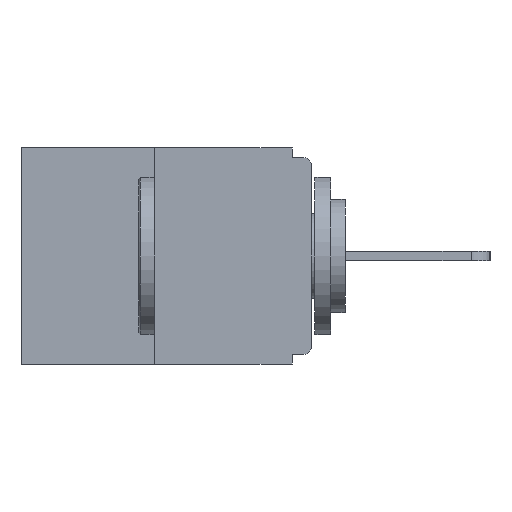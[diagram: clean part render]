
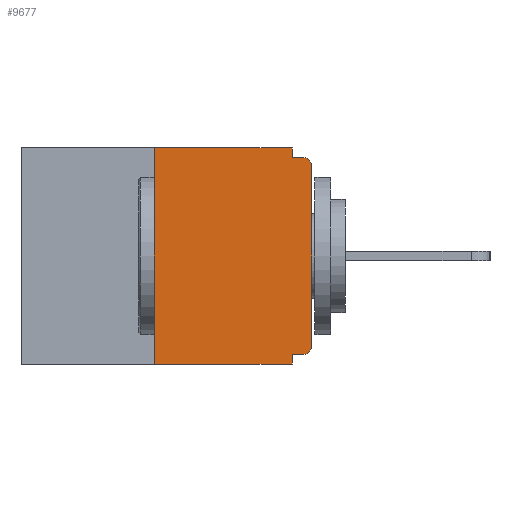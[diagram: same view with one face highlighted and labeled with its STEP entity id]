
A CAD part, left-side view. The second image highlights one B-rep face of the part: STEP entity #9677.
In plain terms, the highlighted planar face has unit normal (-1, 0, 0).
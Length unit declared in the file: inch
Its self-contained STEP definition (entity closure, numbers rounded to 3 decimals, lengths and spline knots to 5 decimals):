
#5 = VECTOR ( 'NONE', #2524, 39.37008 ) ;
#201 = VECTOR ( 'NONE', #8029, 39.37008 ) ;
#351 = EDGE_LOOP ( 'NONE', ( #2896, #9992, #2501, #7942, #8920, #2768, #10894, #2540, #6096, #4621 ) ) ;
#425 = LINE ( 'NONE', #11037, #5 ) ;
#451 = DIRECTION ( 'NONE',  ( 0., -1., 0. ) ) ;
#469 = FACE_OUTER_BOUND ( 'NONE', #351, .T. ) ;
#654 = CARTESIAN_POINT ( 'NONE',  ( 0., 0., -0.328 ) ) ;
#752 = VECTOR ( 'NONE', #10732, 39.37008 ) ;
#760 = VERTEX_POINT ( 'NONE', #10775 ) ;
#823 = EDGE_CURVE ( 'NONE', #9894, #8140, #9922, .T. ) ;
#827 = VERTEX_POINT ( 'NONE', #8096 ) ;
#910 = DIRECTION ( 'NONE',  ( 0., 0., -1. ) ) ;
#939 = VECTOR ( 'NONE', #451, 39.37008 ) ;
#1081 = AXIS2_PLACEMENT_3D ( 'NONE', #4281, #9127, #6223 ) ;
#1718 = CARTESIAN_POINT ( 'NONE',  ( 0., 0.015, -0.313 ) ) ;
#1772 = EDGE_CURVE ( 'NONE', #8972, #7027, #8194, .T. ) ;
#1897 = VERTEX_POINT ( 'NONE', #8373 ) ;
#1944 = AXIS2_PLACEMENT_3D ( 'NONE', #9437, #6791, #910 ) ;
#2027 = EDGE_CURVE ( 'NONE', #760, #12217, #6816, .T. ) ;
#2048 = DIRECTION ( 'NONE',  ( 0., -1., 0. ) ) ;
#2071 = CARTESIAN_POINT ( 'NONE',  ( 0., 0., -0.03 ) ) ;
#2501 = ORIENTED_EDGE ( 'NONE', *, *, #10369, .T. ) ;
#2524 = DIRECTION ( 'NONE',  ( 0., 0., 1. ) ) ;
#2540 = ORIENTED_EDGE ( 'NONE', *, *, #11841, .T. ) ;
#2617 = EDGE_CURVE ( 'NONE', #5414, #9894, #5412, .T. ) ;
#2636 = LINE ( 'NONE', #6466, #2879 ) ;
#2768 = ORIENTED_EDGE ( 'NONE', *, *, #11799, .T. ) ;
#2879 = VECTOR ( 'NONE', #5528, 39.37008 ) ;
#2896 = ORIENTED_EDGE ( 'NONE', *, *, #2027, .F. ) ;
#3311 = DIRECTION ( 'NONE',  ( -1., 0., 0. ) ) ;
#3474 = PLANE ( 'NONE',  #1081 ) ;
#3995 = LINE ( 'NONE', #8959, #752 ) ;
#4281 = CARTESIAN_POINT ( 'NONE',  ( 0., 0.46, 0. ) ) ;
#4326 = CARTESIAN_POINT ( 'NONE',  ( 0., 0., -0.015 ) ) ;
#4356 = AXIS2_PLACEMENT_3D ( 'NONE', #1718, #3311, #10868 ) ;
#4469 = DIRECTION ( 'NONE',  ( 0., 1., 0. ) ) ;
#4621 = ORIENTED_EDGE ( 'NONE', *, *, #6938, .F. ) ;
#4747 = CARTESIAN_POINT ( 'NONE',  ( 0., 0.031, -0.015 ) ) ;
#5168 = CARTESIAN_POINT ( 'NONE',  ( 0., 0.015, -0.328 ) ) ;
#5350 = CARTESIAN_POINT ( 'NONE',  ( 0., 0., 0. ) ) ;
#5412 = LINE ( 'NONE', #654, #9144 ) ;
#5414 = VERTEX_POINT ( 'NONE', #5168 ) ;
#5528 = DIRECTION ( 'NONE',  ( 0., 0., -1. ) ) ;
#5987 = CARTESIAN_POINT ( 'NONE',  ( 0., 0.031, -0.343 ) ) ;
#6096 = ORIENTED_EDGE ( 'NONE', *, *, #1772, .F. ) ;
#6223 = DIRECTION ( 'NONE',  ( 0., 0., -1. ) ) ;
#6466 = CARTESIAN_POINT ( 'NONE',  ( 0., 0.031, 0. ) ) ;
#6747 = CIRCLE ( 'NONE', #1944, 0.015 ) ;
#6791 = DIRECTION ( 'NONE',  ( -1., 0., 0. ) ) ;
#6816 = LINE ( 'NONE', #7685, #7337 ) ;
#6938 = EDGE_CURVE ( 'NONE', #12217, #8972, #2636, .T. ) ;
#7027 = VERTEX_POINT ( 'NONE', #11209 ) ;
#7337 = VECTOR ( 'NONE', #2048, 39.37008 ) ;
#7685 = CARTESIAN_POINT ( 'NONE',  ( 0., 0.46, 0. ) ) ;
#7908 = DIRECTION ( 'NONE',  ( 0., 0., -1. ) ) ;
#7942 = ORIENTED_EDGE ( 'NONE', *, *, #823, .F. ) ;
#8029 = DIRECTION ( 'NONE',  ( 0., 0., 1. ) ) ;
#8096 = CARTESIAN_POINT ( 'NONE',  ( 0., 0.25, -0.343 ) ) ;
#8140 = VERTEX_POINT ( 'NONE', #10913 ) ;
#8194 = LINE ( 'NONE', #4326, #939 ) ;
#8373 = CARTESIAN_POINT ( 'NONE',  ( 0., 0., -0.313 ) ) ;
#8844 = CARTESIAN_POINT ( 'NONE',  ( 0., 0.031, -0.328 ) ) ;
#8920 = ORIENTED_EDGE ( 'NONE', *, *, #2617, .F. ) ;
#8959 = CARTESIAN_POINT ( 'NONE',  ( 0., 0.46, -0.343 ) ) ;
#8972 = VERTEX_POINT ( 'NONE', #4747 ) ;
#9115 = CIRCLE ( 'NONE', #4356, 0.015 ) ;
#9127 = DIRECTION ( 'NONE',  ( 1., 0., 0. ) ) ;
#9143 = EDGE_CURVE ( 'NONE', #827, #760, #425, .T. ) ;
#9144 = VECTOR ( 'NONE', #4469, 39.37008 ) ;
#9437 = CARTESIAN_POINT ( 'NONE',  ( 0., 0.015, -0.03 ) ) ;
#9639 = EDGE_CURVE ( 'NONE', #1897, #11198, #11987, .T. ) ;
#9677 = ADVANCED_FACE ( 'NONE', ( #469 ), #3474, .F. ) ;
#9894 = VERTEX_POINT ( 'NONE', #8844 ) ;
#9922 = LINE ( 'NONE', #5987, #11146 ) ;
#9992 = ORIENTED_EDGE ( 'NONE', *, *, #9143, .F. ) ;
#10035 = CARTESIAN_POINT ( 'NONE',  ( 0., 0.031, 0. ) ) ;
#10369 = EDGE_CURVE ( 'NONE', #827, #8140, #3995, .T. ) ;
#10732 = DIRECTION ( 'NONE',  ( 0., -1., 0. ) ) ;
#10775 = CARTESIAN_POINT ( 'NONE',  ( 0., 0.25, 0. ) ) ;
#10868 = DIRECTION ( 'NONE',  ( 0., 0., -1. ) ) ;
#10894 = ORIENTED_EDGE ( 'NONE', *, *, #9639, .T. ) ;
#10913 = CARTESIAN_POINT ( 'NONE',  ( 0., 0.031, -0.343 ) ) ;
#11037 = CARTESIAN_POINT ( 'NONE',  ( 0., 0.25, 0. ) ) ;
#11146 = VECTOR ( 'NONE', #7908, 39.37008 ) ;
#11198 = VERTEX_POINT ( 'NONE', #2071 ) ;
#11209 = CARTESIAN_POINT ( 'NONE',  ( 0., 0.015, -0.015 ) ) ;
#11799 = EDGE_CURVE ( 'NONE', #5414, #1897, #9115, .T. ) ;
#11841 = EDGE_CURVE ( 'NONE', #11198, #7027, #6747, .T. ) ;
#11987 = LINE ( 'NONE', #5350, #201 ) ;
#12217 = VERTEX_POINT ( 'NONE', #10035 ) ;
